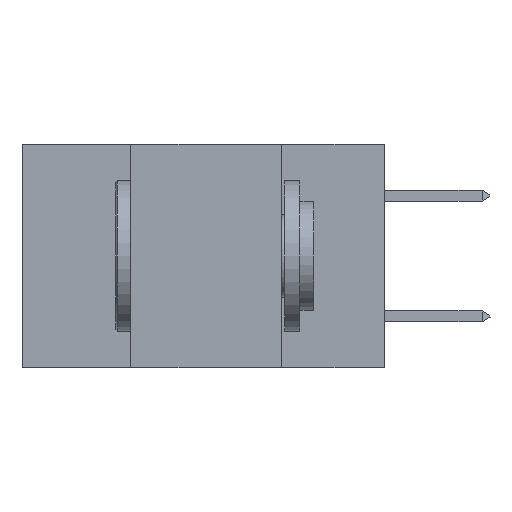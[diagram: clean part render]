
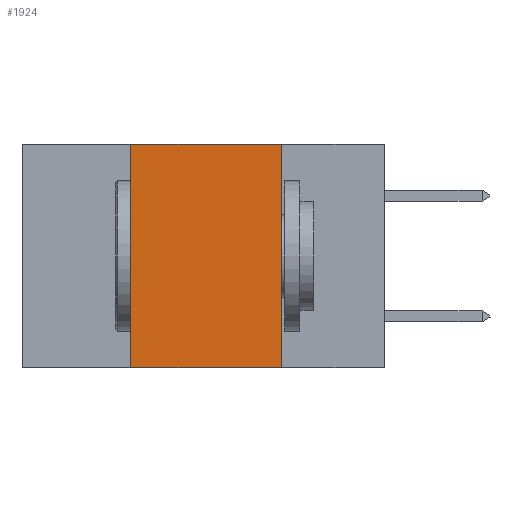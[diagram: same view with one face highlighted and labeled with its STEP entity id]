
A CAD part, left-side view. The second image highlights one B-rep face of the part: STEP entity #1924.
In plain terms, the highlighted planar face has unit normal (-1, 0, 0).
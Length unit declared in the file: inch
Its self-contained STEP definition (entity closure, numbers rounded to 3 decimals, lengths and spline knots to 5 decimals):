
#632 = VERTEX_POINT ( 'NONE', #3342 ) ;
#1924 = ADVANCED_FACE ( 'NONE', ( #19931 ), #10057, .F. ) ;
#2096 = DIRECTION ( 'NONE',  ( 0., -1., 0. ) ) ;
#2539 = CARTESIAN_POINT ( 'NONE',  ( 0., 0.6, 0. ) ) ;
#2646 = AXIS2_PLACEMENT_3D ( 'NONE', #30502, #23580, #16659 ) ;
#3342 = CARTESIAN_POINT ( 'NONE',  ( 0., 0.17, -0.37 ) ) ;
#4927 = CARTESIAN_POINT ( 'NONE',  ( 0., 0.42, 0. ) ) ;
#7008 = CARTESIAN_POINT ( 'NONE',  ( 0., 0.42, -0.37 ) ) ;
#7319 = VERTEX_POINT ( 'NONE', #24229 ) ;
#8479 = DIRECTION ( 'NONE',  ( 0., 0., 1. ) ) ;
#10057 = PLANE ( 'NONE',  #2646 ) ;
#16659 = DIRECTION ( 'NONE',  ( 0., 0., -1. ) ) ;
#18354 = VECTOR ( 'NONE', #2096, 39.37008 ) ;
#19931 = FACE_OUTER_BOUND ( 'NONE', #36311, .T. ) ;
#23580 = DIRECTION ( 'NONE',  ( 1., 0., 0. ) ) ;
#24229 = CARTESIAN_POINT ( 'NONE',  ( 0., 0.42, 0. ) ) ;
#24963 = EDGE_CURVE ( 'NONE', #41140, #632, #37870, .T. ) ;
#25214 = ORIENTED_EDGE ( 'NONE', *, *, #36032, .F. ) ;
#25360 = VECTOR ( 'NONE', #30539, 39.37008 ) ;
#26241 = LINE ( 'NONE', #2539, #18354 ) ;
#26976 = CARTESIAN_POINT ( 'NONE',  ( 0., 0.17, 0. ) ) ;
#27058 = ORIENTED_EDGE ( 'NONE', *, *, #33564, .F. ) ;
#28085 = LINE ( 'NONE', #4927, #29634 ) ;
#28263 = EDGE_CURVE ( 'NONE', #41140, #7319, #28085, .T. ) ;
#28496 = ORIENTED_EDGE ( 'NONE', *, *, #28263, .F. ) ;
#28920 = VECTOR ( 'NONE', #43027, 39.37008 ) ;
#29634 = VECTOR ( 'NONE', #8479, 39.37008 ) ;
#30502 = CARTESIAN_POINT ( 'NONE',  ( 0., 0.6, 0. ) ) ;
#30539 = DIRECTION ( 'NONE',  ( 0., 0., -1. ) ) ;
#31162 = LINE ( 'NONE', #26976, #25360 ) ;
#33564 = EDGE_CURVE ( 'NONE', #40018, #632, #31162, .T. ) ;
#34902 = ORIENTED_EDGE ( 'NONE', *, *, #24963, .T. ) ;
#34945 = CARTESIAN_POINT ( 'NONE',  ( 0., 0.17, 0. ) ) ;
#36032 = EDGE_CURVE ( 'NONE', #7319, #40018, #26241, .T. ) ;
#36311 = EDGE_LOOP ( 'NONE', ( #27058, #25214, #28496, #34902 ) ) ;
#37870 = LINE ( 'NONE', #42748, #28920 ) ;
#40018 = VERTEX_POINT ( 'NONE', #34945 ) ;
#41140 = VERTEX_POINT ( 'NONE', #7008 ) ;
#42748 = CARTESIAN_POINT ( 'NONE',  ( 0., 0.6, -0.37 ) ) ;
#43027 = DIRECTION ( 'NONE',  ( 0., -1., 0. ) ) ;
